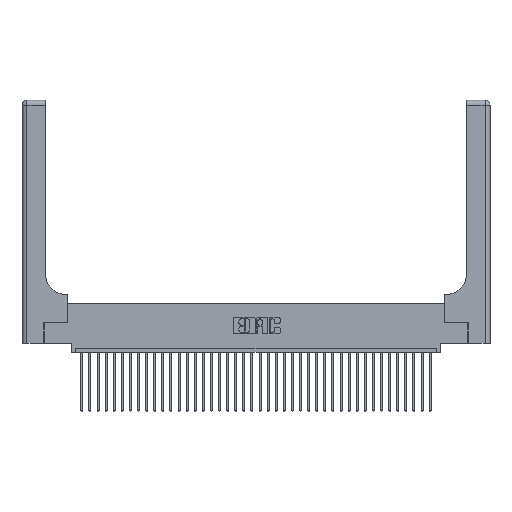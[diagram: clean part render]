
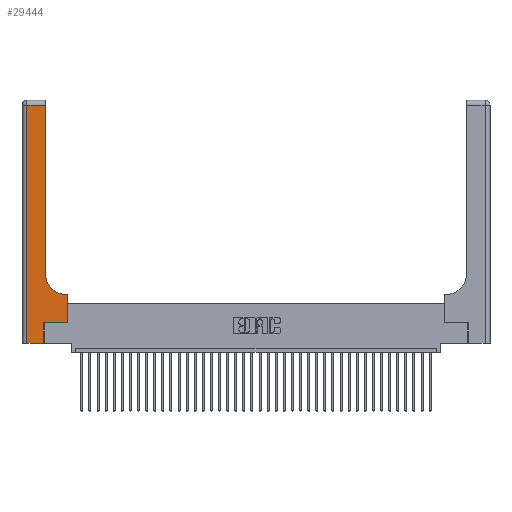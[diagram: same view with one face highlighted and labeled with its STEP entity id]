
A CAD part, top view. The second image highlights one B-rep face of the part: STEP entity #29444.
In plain terms, the highlighted planar face has unit normal (0, 0, 1).
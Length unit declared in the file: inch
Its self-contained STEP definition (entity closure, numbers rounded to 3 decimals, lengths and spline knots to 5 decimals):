
#61 = CIRCLE ( 'NONE', #30436, 0.25 ) ;
#169 = ORIENTED_EDGE ( 'NONE', *, *, #26645, .T. ) ;
#443 = CARTESIAN_POINT ( 'NONE',  ( 0.269, 0.25, 0.37 ) ) ;
#583 = CARTESIAN_POINT ( 'NONE',  ( 0., 0., 0.37 ) ) ;
#1433 = DIRECTION ( 'NONE',  ( 1., 0., 0. ) ) ;
#2172 = CARTESIAN_POINT ( 'NONE',  ( 0., 2.94, 0.37 ) ) ;
#2405 = EDGE_CURVE ( 'NONE', #24039, #25828, #20891, .T. ) ;
#3843 = CARTESIAN_POINT ( 'NONE',  ( 0.269, 0.25, 0.37 ) ) ;
#4041 = FACE_OUTER_BOUND ( 'NONE', #28374, .T. ) ;
#4058 = EDGE_CURVE ( 'NONE', #28799, #4226, #61, .T. ) ;
#4226 = VERTEX_POINT ( 'NONE', #20220 ) ;
#5531 = VECTOR ( 'NONE', #6450, 39.37008 ) ;
#6220 = LINE ( 'NONE', #8007, #24225 ) ;
#6294 = VERTEX_POINT ( 'NONE', #28247 ) ;
#6384 = DIRECTION ( 'NONE',  ( 1., 0., 0. ) ) ;
#6450 = DIRECTION ( 'NONE',  ( 0., 1., 0. ) ) ;
#6975 = DIRECTION ( 'NONE',  ( -1., 0., 0. ) ) ;
#7739 = ORIENTED_EDGE ( 'NONE', *, *, #14412, .T. ) ;
#7749 = CARTESIAN_POINT ( 'NONE',  ( 0.06, 2.94, 0.37 ) ) ;
#7758 = LINE ( 'NONE', #443, #25732 ) ;
#7920 = DIRECTION ( 'NONE',  ( -1., 0., 0. ) ) ;
#8007 = CARTESIAN_POINT ( 'NONE',  ( 0.2915, 3., 0.37 ) ) ;
#8461 = EDGE_CURVE ( 'NONE', #26074, #29964, #22532, .T. ) ;
#9410 = EDGE_CURVE ( 'NONE', #25828, #6294, #7758, .T. ) ;
#10156 = LINE ( 'NONE', #583, #20262 ) ;
#10366 = CARTESIAN_POINT ( 'NONE',  ( 0.2915, 0.6, 0.37 ) ) ;
#11101 = AXIS2_PLACEMENT_3D ( 'NONE', #11529, #31276, #17420 ) ;
#11529 = CARTESIAN_POINT ( 'NONE',  ( 0., 3., 0.37 ) ) ;
#11891 = VECTOR ( 'NONE', #6975, 39.37008 ) ;
#12730 = LINE ( 'NONE', #10366, #13231 ) ;
#12885 = CARTESIAN_POINT ( 'NONE',  ( 0.269, 0., 0.37 ) ) ;
#12998 = EDGE_CURVE ( 'NONE', #29964, #24730, #13051, .T. ) ;
#13051 = LINE ( 'NONE', #37137, #28292 ) ;
#13231 = VECTOR ( 'NONE', #7920, 39.37008 ) ;
#13610 = ORIENTED_EDGE ( 'NONE', *, *, #4058, .T. ) ;
#14412 = EDGE_CURVE ( 'NONE', #24730, #24039, #10156, .T. ) ;
#15354 = ORIENTED_EDGE ( 'NONE', *, *, #2405, .T. ) ;
#15389 = CARTESIAN_POINT ( 'NONE',  ( 0.2915, 2.94, 0.37 ) ) ;
#15721 = CARTESIAN_POINT ( 'NONE',  ( 0.5415, 0.85, 0.37 ) ) ;
#16146 = DIRECTION ( 'NONE',  ( 0., 1., 0. ) ) ;
#17420 = DIRECTION ( 'NONE',  ( -1., 0., 0. ) ) ;
#17696 = CARTESIAN_POINT ( 'NONE',  ( 0.5415, 0.6, 0.37 ) ) ;
#18307 = CARTESIAN_POINT ( 'NONE',  ( 0.5585, 0.6, 0.37 ) ) ;
#20220 = CARTESIAN_POINT ( 'NONE',  ( 0.2915, 0.85, 0.37 ) ) ;
#20262 = VECTOR ( 'NONE', #32840, 39.37008 ) ;
#20632 = ORIENTED_EDGE ( 'NONE', *, *, #12998, .T. ) ;
#20891 = LINE ( 'NONE', #31275, #35692 ) ;
#21250 = CARTESIAN_POINT ( 'NONE',  ( 0.5585, 0.25, 0.37 ) ) ;
#22532 = LINE ( 'NONE', #2172, #11891 ) ;
#22588 = LINE ( 'NONE', #21250, #5531 ) ;
#22589 = DIRECTION ( 'NONE',  ( 0., 1., 0. ) ) ;
#22626 = EDGE_CURVE ( 'NONE', #4226, #26074, #6220, .T. ) ;
#24039 = VERTEX_POINT ( 'NONE', #12885 ) ;
#24225 = VECTOR ( 'NONE', #22589, 39.37008 ) ;
#24730 = VERTEX_POINT ( 'NONE', #37075 ) ;
#25630 = ORIENTED_EDGE ( 'NONE', *, *, #8461, .T. ) ;
#25732 = VECTOR ( 'NONE', #1433, 39.37008 ) ;
#25828 = VERTEX_POINT ( 'NONE', #3843 ) ;
#25917 = ORIENTED_EDGE ( 'NONE', *, *, #9410, .T. ) ;
#26074 = VERTEX_POINT ( 'NONE', #15389 ) ;
#26645 = EDGE_CURVE ( 'NONE', #6294, #34880, #22588, .T. ) ;
#28152 = DIRECTION ( 'NONE',  ( 0., -1., 0. ) ) ;
#28247 = CARTESIAN_POINT ( 'NONE',  ( 0.5585, 0.25, 0.37 ) ) ;
#28292 = VECTOR ( 'NONE', #28152, 39.37008 ) ;
#28374 = EDGE_LOOP ( 'NONE', ( #31077, #25630, #20632, #7739, #15354, #25917, #169, #33826, #13610 ) ) ;
#28799 = VERTEX_POINT ( 'NONE', #17696 ) ;
#29444 = ADVANCED_FACE ( 'NONE', ( #4041 ), #34227, .F. ) ;
#29964 = VERTEX_POINT ( 'NONE', #7749 ) ;
#30436 = AXIS2_PLACEMENT_3D ( 'NONE', #15721, #30454, #6384 ) ;
#30454 = DIRECTION ( 'NONE',  ( 0., 0., -1. ) ) ;
#31077 = ORIENTED_EDGE ( 'NONE', *, *, #22626, .T. ) ;
#31275 = CARTESIAN_POINT ( 'NONE',  ( 0.269, 0., 0.37 ) ) ;
#31276 = DIRECTION ( 'NONE',  ( 0., 0., -1. ) ) ;
#32840 = DIRECTION ( 'NONE',  ( 1., 0., 0. ) ) ;
#33826 = ORIENTED_EDGE ( 'NONE', *, *, #36709, .T. ) ;
#34227 = PLANE ( 'NONE',  #11101 ) ;
#34880 = VERTEX_POINT ( 'NONE', #18307 ) ;
#35692 = VECTOR ( 'NONE', #16146, 39.37008 ) ;
#36709 = EDGE_CURVE ( 'NONE', #34880, #28799, #12730, .T. ) ;
#37075 = CARTESIAN_POINT ( 'NONE',  ( 0.06, 0., 0.37 ) ) ;
#37137 = CARTESIAN_POINT ( 'NONE',  ( 0.06, 3., 0.37 ) ) ;
